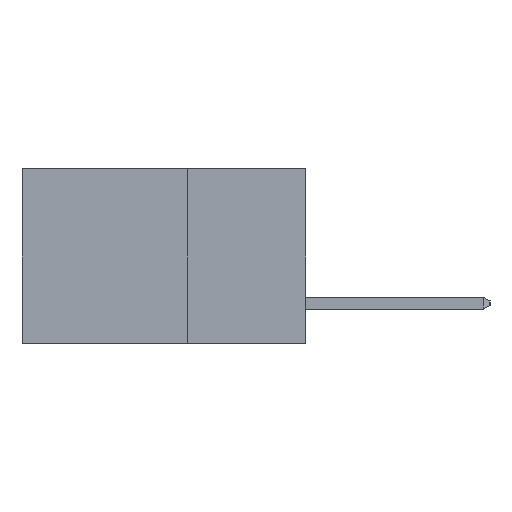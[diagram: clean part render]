
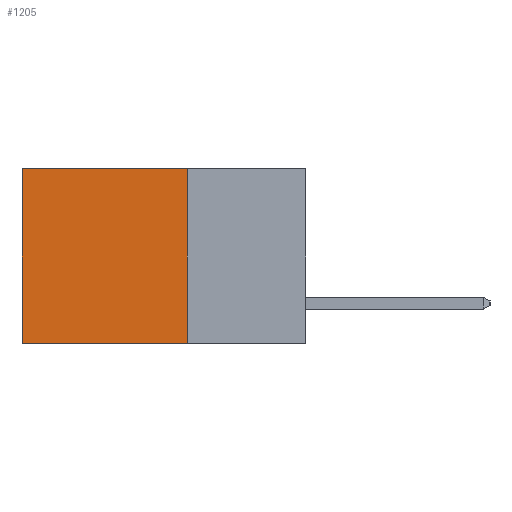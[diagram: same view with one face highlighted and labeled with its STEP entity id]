
A CAD part, left-side view. The second image highlights one B-rep face of the part: STEP entity #1205.
In plain terms, the highlighted planar face has unit normal (-1, 0, 0).
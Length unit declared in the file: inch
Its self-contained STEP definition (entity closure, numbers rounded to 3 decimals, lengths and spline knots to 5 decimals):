
#84 = DIRECTION ( 'NONE',  ( 0., 0., -1. ) ) ;
#892 = CARTESIAN_POINT ( 'NONE',  ( 0.2615, 0.6, 0. ) ) ;
#943 = LINE ( 'NONE', #3935, #4452 ) ;
#1205 = ADVANCED_FACE ( 'NONE', ( #6303 ), #7749, .F. ) ;
#1453 = ORIENTED_EDGE ( 'NONE', *, *, #6573, .F. ) ;
#1509 = DIRECTION ( 'NONE',  ( 0., 1., 0. ) ) ;
#1880 = DIRECTION ( 'NONE',  ( 0., 0., -1. ) ) ;
#2150 = CARTESIAN_POINT ( 'NONE',  ( 0.2615, 0.25, -0.37 ) ) ;
#2160 = DIRECTION ( 'NONE',  ( 1., 0., 0. ) ) ;
#2339 = VECTOR ( 'NONE', #7814, 39.37008 ) ;
#2399 = EDGE_CURVE ( 'NONE', #4768, #6894, #7518, .T. ) ;
#2579 = EDGE_CURVE ( 'NONE', #4768, #5088, #943, .T. ) ;
#2597 = ORIENTED_EDGE ( 'NONE', *, *, #2579, .F. ) ;
#2784 = CARTESIAN_POINT ( 'NONE',  ( 0.2615, 0.6, -0.37 ) ) ;
#2892 = CARTESIAN_POINT ( 'NONE',  ( 0.2615, 0.25, -0.37 ) ) ;
#3185 = VECTOR ( 'NONE', #4844, 39.37008 ) ;
#3935 = CARTESIAN_POINT ( 'NONE',  ( 0.2615, 0.25, -0.37 ) ) ;
#4407 = LINE ( 'NONE', #8308, #2339 ) ;
#4452 = VECTOR ( 'NONE', #84, 39.37008 ) ;
#4754 = VERTEX_POINT ( 'NONE', #2784 ) ;
#4768 = VERTEX_POINT ( 'NONE', #4808 ) ;
#4808 = CARTESIAN_POINT ( 'NONE',  ( 0.2615, 0.25, 0. ) ) ;
#4818 = CARTESIAN_POINT ( 'NONE',  ( 0.2615, 0.25, -0.37 ) ) ;
#4844 = DIRECTION ( 'NONE',  ( 0., 1., 0. ) ) ;
#5037 = LINE ( 'NONE', #4818, #3185 ) ;
#5080 = EDGE_LOOP ( 'NONE', ( #6240, #1453, #2597, #6255 ) ) ;
#5088 = VERTEX_POINT ( 'NONE', #2892 ) ;
#5718 = VECTOR ( 'NONE', #1509, 39.37008 ) ;
#5835 = EDGE_CURVE ( 'NONE', #6894, #4754, #4407, .T. ) ;
#6240 = ORIENTED_EDGE ( 'NONE', *, *, #5835, .T. ) ;
#6255 = ORIENTED_EDGE ( 'NONE', *, *, #2399, .T. ) ;
#6303 = FACE_OUTER_BOUND ( 'NONE', #5080, .T. ) ;
#6573 = EDGE_CURVE ( 'NONE', #5088, #4754, #5037, .T. ) ;
#6653 = CARTESIAN_POINT ( 'NONE',  ( 0.2615, 0.25, 0. ) ) ;
#6894 = VERTEX_POINT ( 'NONE', #892 ) ;
#7518 = LINE ( 'NONE', #6653, #5718 ) ;
#7749 = PLANE ( 'NONE',  #8470 ) ;
#7814 = DIRECTION ( 'NONE',  ( 0., 0., -1. ) ) ;
#8308 = CARTESIAN_POINT ( 'NONE',  ( 0.2615, 0.6, -0.37 ) ) ;
#8470 = AXIS2_PLACEMENT_3D ( 'NONE', #2150, #2160, #1880 ) ;
